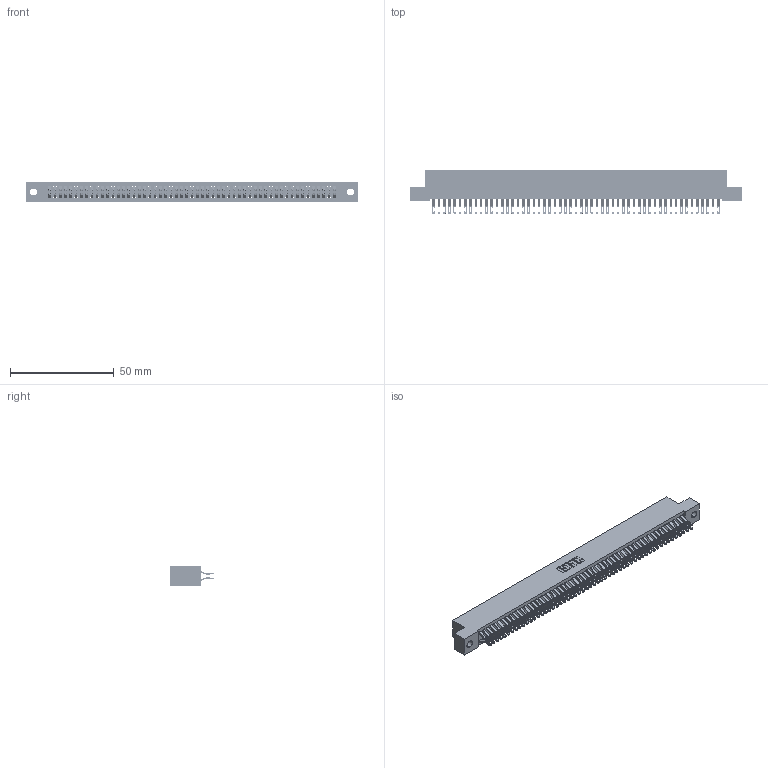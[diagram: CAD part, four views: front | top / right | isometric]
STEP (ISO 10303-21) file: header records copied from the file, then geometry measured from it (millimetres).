
FILE_DESCRIPTION (( 'STEP AP203' ), '1' );
FILE_NAME ('392-110-555-202.STEP', '2019-10-09T23:55:06', ( '' ), ( '' ), 'SwSTEP 2.0', 'SolidWorks 2016', '' );
FILE_SCHEMA (( 'CONFIG_CONTROL_DESIGN' ));
Length unit declared in the file: inch
Products named in the file (3): 342 Part_.128 Slot; 345-292-001_555 Tail; 392-110-555-202
Assembly tree (111 placements, depth 2):
  392-110-555-202
    342 Part_.128 Slot
    345-292-001_555 Tail  x110
Bounding box: 160.02 x 21.47 x 9.4 mm (x, y, z)
Volume: 14692.9 mm3; surface area: 25060.4 mm2
Topology: 111 solids, 111 shells, 6494 faces, 20441 edges, 13626 vertices
Faces by surface type: plane 3810, cylinder 2684
Entity records: 34031 total; most frequent: CARTESIAN_POINT 5660, ORIENTED_EDGE 5566, DIRECTION 4783, EDGE_CURVE 2783, VECTOR 2635, LINE 2635, VERTEX_POINT 1854, AXIS2_PLACEMENT_3D 1074
